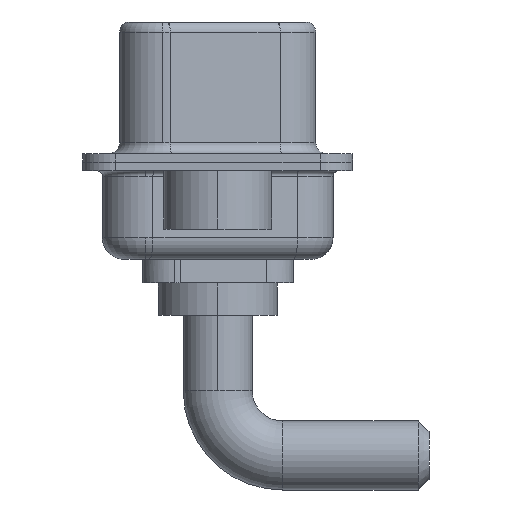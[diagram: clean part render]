
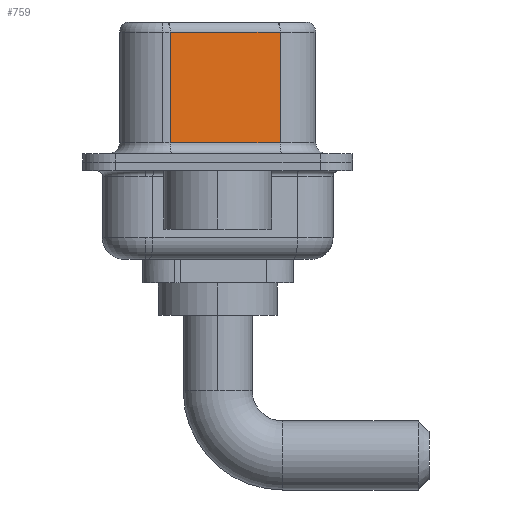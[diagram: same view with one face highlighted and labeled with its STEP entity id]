
A CAD part, left-side view. The second image highlights one B-rep face of the part: STEP entity #759.
In plain terms, the highlighted planar face has unit normal (-0.985, -0.174, 0).
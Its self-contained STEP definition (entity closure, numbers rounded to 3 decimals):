
#171 = PLANE ( 'NONE',  #1502 ) ;
#444 = CARTESIAN_POINT ( 'NONE',  ( 4.58, -2.897, 6.52 ) ) ;
#695 = CARTESIAN_POINT ( 'NONE',  ( 4.58, -2.897, 0.9 ) ) ;
#759 = ADVANCED_FACE ( 'NONE', ( #14861 ), #171, .F. ) ;
#857 = VECTOR ( 'NONE', #11631, 1000. ) ;
#1502 = AXIS2_PLACEMENT_3D ( 'NONE', #6438, #11395, #3766 ) ;
#1726 = DIRECTION ( 'NONE',  ( 0., 0., -1. ) ) ;
#1727 = CARTESIAN_POINT ( 'NONE',  ( 4.58, -2.897, 0.9 ) ) ;
#2185 = LINE ( 'NONE', #15802, #14047 ) ;
#2464 = EDGE_CURVE ( 'NONE', #3209, #12968, #9925, .T. ) ;
#2514 = VECTOR ( 'NONE', #7927, 1000. ) ;
#2944 = CARTESIAN_POINT ( 'NONE',  ( 3.68, 2.203, 0.9 ) ) ;
#3209 = VERTEX_POINT ( 'NONE', #4581 ) ;
#3353 = EDGE_LOOP ( 'NONE', ( #4985, #3428, #13668, #6169 ) ) ;
#3428 = ORIENTED_EDGE ( 'NONE', *, *, #12996, .T. ) ;
#3766 = DIRECTION ( 'NONE',  ( -0.174, 0.985, 0. ) ) ;
#4581 = CARTESIAN_POINT ( 'NONE',  ( 4.58, -2.897, 6.02 ) ) ;
#4985 = ORIENTED_EDGE ( 'NONE', *, *, #2464, .F. ) ;
#5831 = DIRECTION ( 'NONE',  ( -0.174, 0.985, 0. ) ) ;
#6169 = ORIENTED_EDGE ( 'NONE', *, *, #10776, .T. ) ;
#6438 = CARTESIAN_POINT ( 'NONE',  ( 4.58, -2.897, 6.52 ) ) ;
#7927 = DIRECTION ( 'NONE',  ( 0., 0., -1. ) ) ;
#9925 = LINE ( 'NONE', #444, #2514 ) ;
#10704 = CARTESIAN_POINT ( 'NONE',  ( 4.58, -2.897, 6.02 ) ) ;
#10713 = VERTEX_POINT ( 'NONE', #2944 ) ;
#10776 = EDGE_CURVE ( 'NONE', #10713, #12968, #12866, .T. ) ;
#11395 = DIRECTION ( 'NONE',  ( 0.985, 0.174, 0. ) ) ;
#11631 = DIRECTION ( 'NONE',  ( 0.174, -0.985, 0. ) ) ;
#12866 = LINE ( 'NONE', #1727, #857 ) ;
#12968 = VERTEX_POINT ( 'NONE', #695 ) ;
#12996 = EDGE_CURVE ( 'NONE', #3209, #14942, #13160, .T. ) ;
#13160 = LINE ( 'NONE', #10704, #14154 ) ;
#13668 = ORIENTED_EDGE ( 'NONE', *, *, #14581, .T. ) ;
#14047 = VECTOR ( 'NONE', #1726, 1000. ) ;
#14154 = VECTOR ( 'NONE', #5831, 1000. ) ;
#14581 = EDGE_CURVE ( 'NONE', #14942, #10713, #2185, .T. ) ;
#14861 = FACE_OUTER_BOUND ( 'NONE', #3353, .T. ) ;
#14942 = VERTEX_POINT ( 'NONE', #15862 ) ;
#15802 = CARTESIAN_POINT ( 'NONE',  ( 3.68, 2.203, 6.52 ) ) ;
#15862 = CARTESIAN_POINT ( 'NONE',  ( 3.68, 2.203, 6.02 ) ) ;
